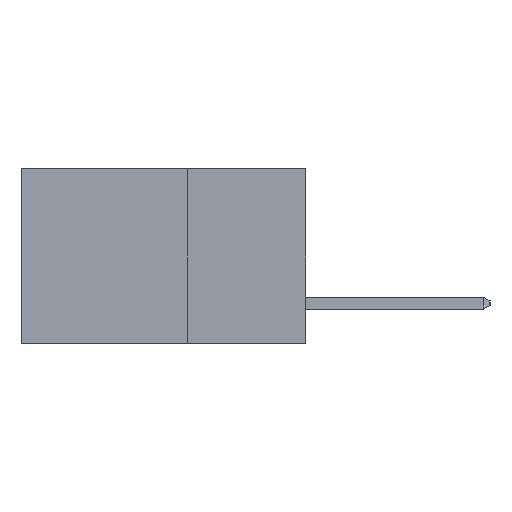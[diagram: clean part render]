
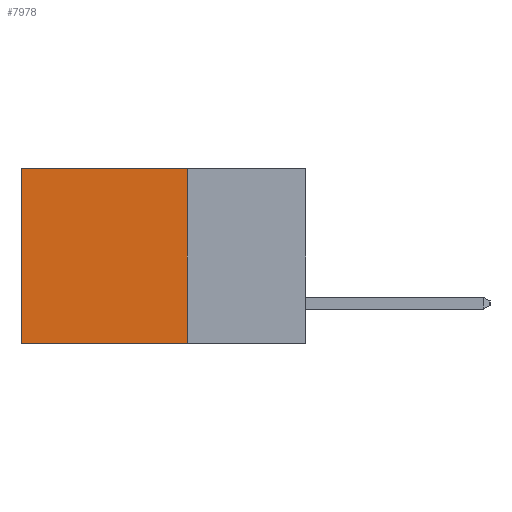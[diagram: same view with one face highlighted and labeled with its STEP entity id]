
A CAD part, left-side view. The second image highlights one B-rep face of the part: STEP entity #7978.
In plain terms, the highlighted planar face has unit normal (-1, 0, 0).
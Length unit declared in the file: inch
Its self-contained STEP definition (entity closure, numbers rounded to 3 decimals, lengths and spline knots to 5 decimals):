
#483 = ORIENTED_EDGE ( 'NONE', *, *, #1878, .F. ) ;
#490 = CARTESIAN_POINT ( 'NONE',  ( 0.2615, 0.6, -0.37 ) ) ;
#506 = PLANE ( 'NONE',  #8995 ) ;
#1415 = CARTESIAN_POINT ( 'NONE',  ( 0.2615, 0.6, 0. ) ) ;
#1482 = VERTEX_POINT ( 'NONE', #5552 ) ;
#1823 = DIRECTION ( 'NONE',  ( 0., 0., -1. ) ) ;
#1878 = EDGE_CURVE ( 'NONE', #1482, #2430, #3353, .T. ) ;
#2128 = CARTESIAN_POINT ( 'NONE',  ( 0.2615, 0.25, -0.37 ) ) ;
#2258 = CARTESIAN_POINT ( 'NONE',  ( 0.2615, 0.6, -0.37 ) ) ;
#2371 = ORIENTED_EDGE ( 'NONE', *, *, #4892, .T. ) ;
#2430 = VERTEX_POINT ( 'NONE', #8386 ) ;
#2574 = EDGE_CURVE ( 'NONE', #1482, #3704, #2920, .T. ) ;
#2735 = DIRECTION ( 'NONE',  ( 0., 1., 0. ) ) ;
#2920 = LINE ( 'NONE', #8274, #9160 ) ;
#2956 = EDGE_LOOP ( 'NONE', ( #2371, #5959, #483, #3786 ) ) ;
#3295 = DIRECTION ( 'NONE',  ( 1., 0., 0. ) ) ;
#3353 = LINE ( 'NONE', #2128, #7321 ) ;
#3523 = VERTEX_POINT ( 'NONE', #490 ) ;
#3704 = VERTEX_POINT ( 'NONE', #1415 ) ;
#3786 = ORIENTED_EDGE ( 'NONE', *, *, #2574, .T. ) ;
#4111 = CARTESIAN_POINT ( 'NONE',  ( 0.2615, 0.25, -0.37 ) ) ;
#4323 = DIRECTION ( 'NONE',  ( 0., 0., -1. ) ) ;
#4892 = EDGE_CURVE ( 'NONE', #3704, #3523, #9529, .T. ) ;
#5552 = CARTESIAN_POINT ( 'NONE',  ( 0.2615, 0.25, 0. ) ) ;
#5959 = ORIENTED_EDGE ( 'NONE', *, *, #9862, .F. ) ;
#6328 = LINE ( 'NONE', #7544, #6576 ) ;
#6576 = VECTOR ( 'NONE', #2735, 39.37008 ) ;
#7057 = VECTOR ( 'NONE', #1823, 39.37008 ) ;
#7109 = FACE_OUTER_BOUND ( 'NONE', #2956, .T. ) ;
#7321 = VECTOR ( 'NONE', #4323, 39.37008 ) ;
#7544 = CARTESIAN_POINT ( 'NONE',  ( 0.2615, 0.25, -0.37 ) ) ;
#7978 = ADVANCED_FACE ( 'NONE', ( #7109 ), #506, .F. ) ;
#8264 = DIRECTION ( 'NONE',  ( 0., 1., 0. ) ) ;
#8274 = CARTESIAN_POINT ( 'NONE',  ( 0.2615, 0.25, 0. ) ) ;
#8386 = CARTESIAN_POINT ( 'NONE',  ( 0.2615, 0.25, -0.37 ) ) ;
#8934 = DIRECTION ( 'NONE',  ( 0., 0., -1. ) ) ;
#8995 = AXIS2_PLACEMENT_3D ( 'NONE', #4111, #3295, #8934 ) ;
#9160 = VECTOR ( 'NONE', #8264, 39.37008 ) ;
#9529 = LINE ( 'NONE', #2258, #7057 ) ;
#9862 = EDGE_CURVE ( 'NONE', #2430, #3523, #6328, .T. ) ;
